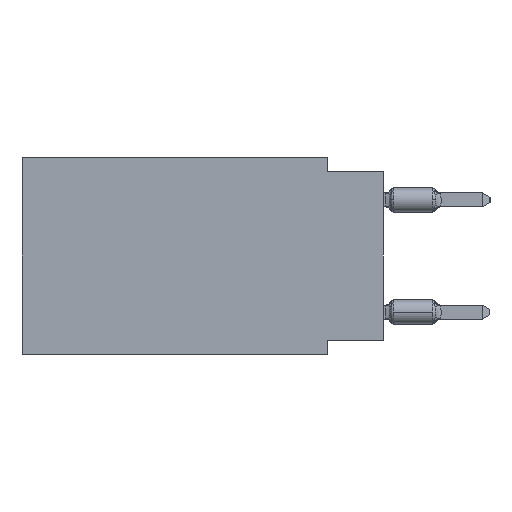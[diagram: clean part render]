
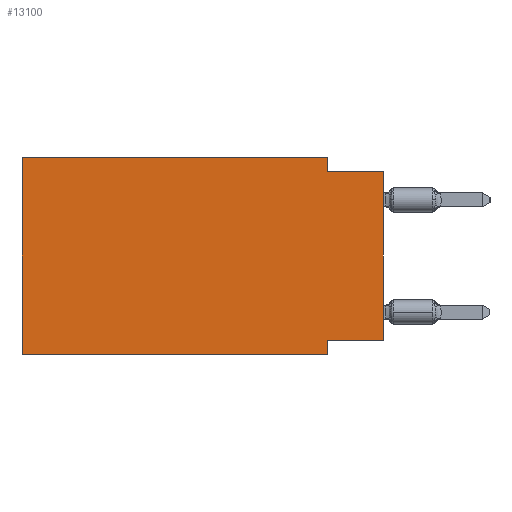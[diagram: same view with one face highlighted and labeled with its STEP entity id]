
A CAD part, left-side view. The second image highlights one B-rep face of the part: STEP entity #13100.
In plain terms, the highlighted planar face has unit normal (-1, 0, 0).
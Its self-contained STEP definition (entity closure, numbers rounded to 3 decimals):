
#457 = VECTOR ( 'NONE', #6013, 1000. ) ;
#535 = CARTESIAN_POINT ( 'NONE',  ( 0., 16.383, -8.89 ) ) ;
#790 = DIRECTION ( 'NONE',  ( 0., -1., 0. ) ) ;
#793 = FACE_OUTER_BOUND ( 'NONE', #37917, .T. ) ;
#1541 = LINE ( 'NONE', #16786, #17330 ) ;
#2032 = CARTESIAN_POINT ( 'NONE',  ( 0., 16.383, 0. ) ) ;
#2922 = VECTOR ( 'NONE', #28783, 1000. ) ;
#3089 = VERTEX_POINT ( 'NONE', #20549 ) ;
#4572 = VERTEX_POINT ( 'NONE', #535 ) ;
#5142 = CARTESIAN_POINT ( 'NONE',  ( 0., 2.54, -8.255 ) ) ;
#5642 = DIRECTION ( 'NONE',  ( 0., 0., -1. ) ) ;
#5819 = DIRECTION ( 'NONE',  ( 0., 1., 0. ) ) ;
#6013 = DIRECTION ( 'NONE',  ( 0., -1., 0. ) ) ;
#6706 = EDGE_CURVE ( 'NONE', #36093, #3089, #13033, .T. ) ;
#7810 = CARTESIAN_POINT ( 'NONE',  ( 0., 16.383, 0. ) ) ;
#8033 = LINE ( 'NONE', #46014, #13718 ) ;
#8286 = CARTESIAN_POINT ( 'NONE',  ( 0., 16.383, 0. ) ) ;
#9509 = CARTESIAN_POINT ( 'NONE',  ( 0., 2.54, -0.635 ) ) ;
#11810 = PLANE ( 'NONE',  #36904 ) ;
#11884 = DIRECTION ( 'NONE',  ( 0., 0., -1. ) ) ;
#13032 = DIRECTION ( 'NONE',  ( 0., 0., 1. ) ) ;
#13033 = LINE ( 'NONE', #28042, #457 ) ;
#13100 = ADVANCED_FACE ( 'NONE', ( #793 ), #11810, .F. ) ;
#13422 = ORIENTED_EDGE ( 'NONE', *, *, #46468, .F. ) ;
#13718 = VECTOR ( 'NONE', #790, 1000. ) ;
#14908 = VERTEX_POINT ( 'NONE', #36932 ) ;
#15092 = VECTOR ( 'NONE', #5819, 1000. ) ;
#15867 = CARTESIAN_POINT ( 'NONE',  ( 0., 2.54, -8.89 ) ) ;
#16098 = ORIENTED_EDGE ( 'NONE', *, *, #25410, .T. ) ;
#16281 = DIRECTION ( 'NONE',  ( 0., 0., -1. ) ) ;
#16294 = LINE ( 'NONE', #7810, #46073 ) ;
#16786 = CARTESIAN_POINT ( 'NONE',  ( 0., 0., 0. ) ) ;
#16890 = VECTOR ( 'NONE', #5642, 1000. ) ;
#17330 = VECTOR ( 'NONE', #13032, 1000. ) ;
#18180 = VERTEX_POINT ( 'NONE', #43011 ) ;
#18345 = EDGE_CURVE ( 'NONE', #14908, #36906, #39997, .T. ) ;
#19616 = ORIENTED_EDGE ( 'NONE', *, *, #33083, .F. ) ;
#20549 = CARTESIAN_POINT ( 'NONE',  ( 0., 0., -0.635 ) ) ;
#23525 = DIRECTION ( 'NONE',  ( 1., 0., 0. ) ) ;
#24573 = ORIENTED_EDGE ( 'NONE', *, *, #31479, .T. ) ;
#24921 = ORIENTED_EDGE ( 'NONE', *, *, #6706, .F. ) ;
#25410 = EDGE_CURVE ( 'NONE', #4572, #18180, #8033, .T. ) ;
#28042 = CARTESIAN_POINT ( 'NONE',  ( 0., 0., -0.635 ) ) ;
#28587 = LINE ( 'NONE', #44032, #15092 ) ;
#28783 = DIRECTION ( 'NONE',  ( 0., -1., 0. ) ) ;
#30367 = LINE ( 'NONE', #15867, #38532 ) ;
#31479 = EDGE_CURVE ( 'NONE', #37113, #3089, #1541, .T. ) ;
#33083 = EDGE_CURVE ( 'NONE', #4572, #14908, #16294, .T. ) ;
#36093 = VERTEX_POINT ( 'NONE', #9509 ) ;
#36128 = LINE ( 'NONE', #39871, #16890 ) ;
#36904 = AXIS2_PLACEMENT_3D ( 'NONE', #8286, #23525, #16281 ) ;
#36906 = VERTEX_POINT ( 'NONE', #45682 ) ;
#36932 = CARTESIAN_POINT ( 'NONE',  ( 0., 16.383, 0. ) ) ;
#37113 = VERTEX_POINT ( 'NONE', #38942 ) ;
#37917 = EDGE_LOOP ( 'NONE', ( #24573, #24921, #43268, #47019, #19616, #16098, #13422, #47641 ) ) ;
#38532 = VECTOR ( 'NONE', #11884, 1000. ) ;
#38664 = VERTEX_POINT ( 'NONE', #5142 ) ;
#38942 = CARTESIAN_POINT ( 'NONE',  ( 0., 0., -8.255 ) ) ;
#39871 = CARTESIAN_POINT ( 'NONE',  ( 0., 2.54, 0. ) ) ;
#39997 = LINE ( 'NONE', #2032, #2922 ) ;
#42512 = DIRECTION ( 'NONE',  ( 0., 0., 1. ) ) ;
#43011 = CARTESIAN_POINT ( 'NONE',  ( 0., 2.54, -8.89 ) ) ;
#43268 = ORIENTED_EDGE ( 'NONE', *, *, #44800, .F. ) ;
#44032 = CARTESIAN_POINT ( 'NONE',  ( 0., 0., -8.255 ) ) ;
#44800 = EDGE_CURVE ( 'NONE', #36906, #36093, #36128, .T. ) ;
#45682 = CARTESIAN_POINT ( 'NONE',  ( 0., 2.54, 0. ) ) ;
#46014 = CARTESIAN_POINT ( 'NONE',  ( 0., 16.383, -8.89 ) ) ;
#46073 = VECTOR ( 'NONE', #42512, 1000. ) ;
#46468 = EDGE_CURVE ( 'NONE', #38664, #18180, #30367, .T. ) ;
#47019 = ORIENTED_EDGE ( 'NONE', *, *, #18345, .F. ) ;
#47641 = ORIENTED_EDGE ( 'NONE', *, *, #48550, .F. ) ;
#48550 = EDGE_CURVE ( 'NONE', #37113, #38664, #28587, .T. ) ;
